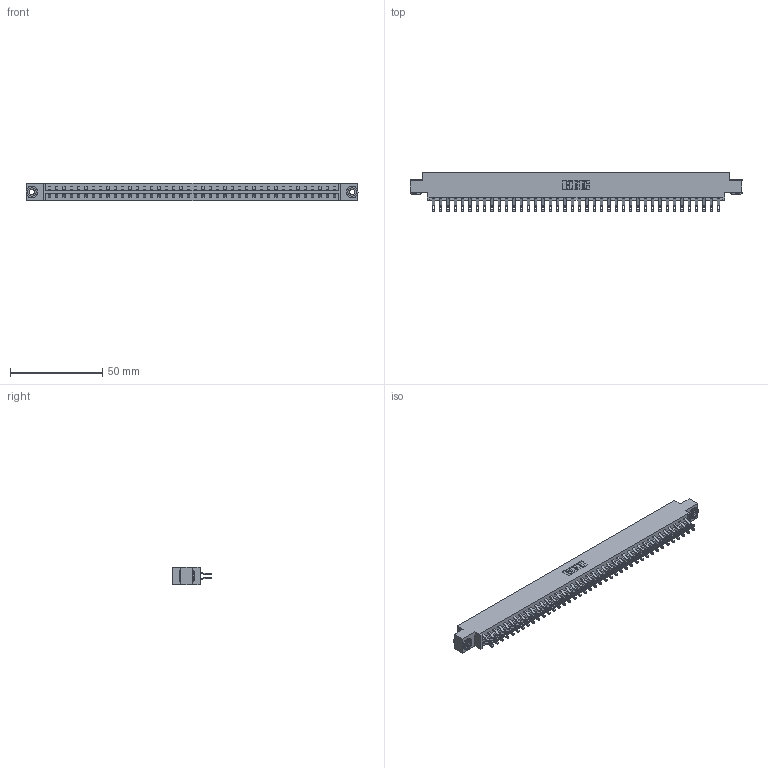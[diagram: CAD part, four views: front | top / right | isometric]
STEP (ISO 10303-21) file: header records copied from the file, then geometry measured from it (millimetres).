
FILE_DESCRIPTION (( 'STEP AP203' ), '1' );
FILE_NAME ('833-080-555-803.STEP', '2020-06-05T22:17:41', ( '' ), ( '' ), 'SwSTEP 2.0', 'SolidWorks 2020', '' );
FILE_SCHEMA (( 'CONFIG_CONTROL_DESIGN' ));
Length unit declared in the file: inch
Products named in the file (4): 833 Part_Offset - .156 Dia - TH; 833-080-555-803; 345-250-002_345-250-002-102; 345-292-001_555 Tail
Assembly tree (83 placements, depth 2):
  833-080-555-803
    833 Part_Offset - .156 Dia - TH
    345-292-001_555 Tail  x80
    345-250-002_345-250-002-102  x2
Bounding box: 180.04 x 21.47 x 9.4 mm (x, y, z)
Volume: 18385.5 mm3; surface area: 23024.3 mm2
Topology: 83 solids, 83 shells, 4796 faces, 15039 edges, 10022 vertices
Faces by surface type: plane 2804, cylinder 1984, cone 8
Entity records: 27100 total; most frequent: CARTESIAN_POINT 4507, ORIENTED_EDGE 4406, DIRECTION 3857, EDGE_CURVE 2203, VECTOR 2031, LINE 2031, VERTEX_POINT 1466, AXIS2_PLACEMENT_3D 913
